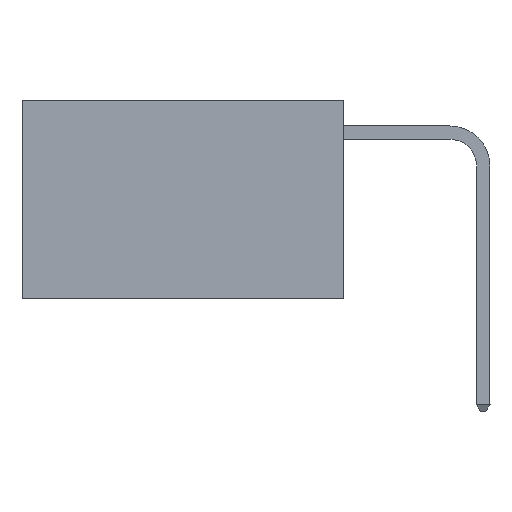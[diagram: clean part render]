
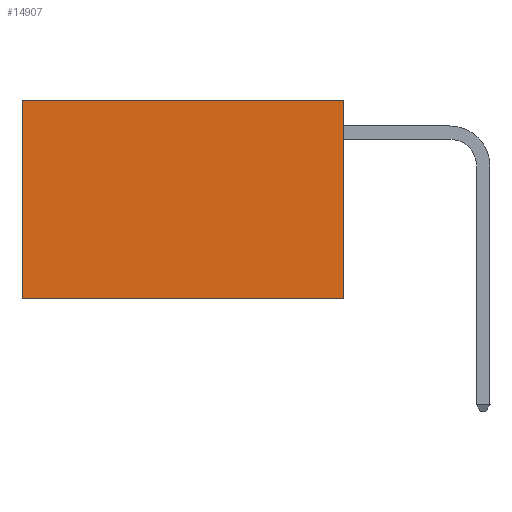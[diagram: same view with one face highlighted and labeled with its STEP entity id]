
A CAD part, left-side view. The second image highlights one B-rep face of the part: STEP entity #14907.
In plain terms, the highlighted planar face has unit normal (-1, 0, 0).
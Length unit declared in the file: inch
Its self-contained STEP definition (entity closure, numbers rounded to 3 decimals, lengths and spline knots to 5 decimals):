
#603 = ORIENTED_EDGE ( 'NONE', *, *, #10272, .F. ) ;
#1100 = VECTOR ( 'NONE', #14791, 39.37008 ) ;
#1592 = LINE ( 'NONE', #4540, #9953 ) ;
#1731 = DIRECTION ( 'NONE',  ( 0., 0., -1. ) ) ;
#2927 = VERTEX_POINT ( 'NONE', #11636 ) ;
#3040 = DIRECTION ( 'NONE',  ( 0., 0., -1. ) ) ;
#3442 = EDGE_LOOP ( 'NONE', ( #10868, #603, #18146, #11902 ) ) ;
#3582 = LINE ( 'NONE', #6535, #19417 ) ;
#3651 = AXIS2_PLACEMENT_3D ( 'NONE', #17160, #11105, #1731 ) ;
#3692 = LINE ( 'NONE', #19867, #7834 ) ;
#4404 = EDGE_CURVE ( 'NONE', #14064, #7557, #3582, .T. ) ;
#4540 = CARTESIAN_POINT ( 'NONE',  ( 0.2625, 0.6, 0. ) ) ;
#5537 = CARTESIAN_POINT ( 'NONE',  ( 0.2625, 0., -0.37 ) ) ;
#6077 = DIRECTION ( 'NONE',  ( 0., 0., -1. ) ) ;
#6426 = PLANE ( 'NONE',  #3651 ) ;
#6535 = CARTESIAN_POINT ( 'NONE',  ( 0.2625, 0., 0. ) ) ;
#7557 = VERTEX_POINT ( 'NONE', #8284 ) ;
#7827 = VERTEX_POINT ( 'NONE', #13430 ) ;
#7834 = VECTOR ( 'NONE', #6077, 39.37008 ) ;
#8284 = CARTESIAN_POINT ( 'NONE',  ( 0.2625, 0.6, 0. ) ) ;
#9953 = VECTOR ( 'NONE', #3040, 39.37008 ) ;
#10272 = EDGE_CURVE ( 'NONE', #2927, #7827, #17629, .T. ) ;
#10868 = ORIENTED_EDGE ( 'NONE', *, *, #20053, .T. ) ;
#11105 = DIRECTION ( 'NONE',  ( 1., 0., 0. ) ) ;
#11585 = DIRECTION ( 'NONE',  ( 0., 1., 0. ) ) ;
#11636 = CARTESIAN_POINT ( 'NONE',  ( 0.2625, 0., -0.37 ) ) ;
#11902 = ORIENTED_EDGE ( 'NONE', *, *, #4404, .T. ) ;
#13430 = CARTESIAN_POINT ( 'NONE',  ( 0.2625, 0.6, -0.37 ) ) ;
#14064 = VERTEX_POINT ( 'NONE', #16576 ) ;
#14791 = DIRECTION ( 'NONE',  ( 0., 1., 0. ) ) ;
#14907 = ADVANCED_FACE ( 'NONE', ( #15731 ), #6426, .F. ) ;
#15731 = FACE_OUTER_BOUND ( 'NONE', #3442, .T. ) ;
#16576 = CARTESIAN_POINT ( 'NONE',  ( 0.2625, 0., 0. ) ) ;
#17160 = CARTESIAN_POINT ( 'NONE',  ( 0.2625, 0., 0. ) ) ;
#17629 = LINE ( 'NONE', #5537, #1100 ) ;
#18012 = EDGE_CURVE ( 'NONE', #14064, #2927, #3692, .T. ) ;
#18146 = ORIENTED_EDGE ( 'NONE', *, *, #18012, .F. ) ;
#19417 = VECTOR ( 'NONE', #11585, 39.37008 ) ;
#19867 = CARTESIAN_POINT ( 'NONE',  ( 0.2625, 0., 0. ) ) ;
#20053 = EDGE_CURVE ( 'NONE', #7557, #7827, #1592, .T. ) ;
